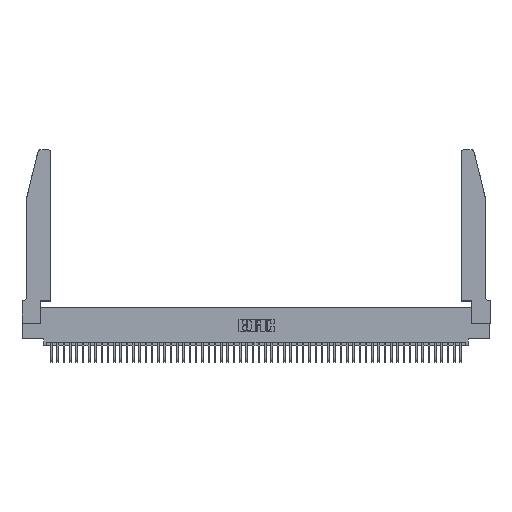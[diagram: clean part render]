
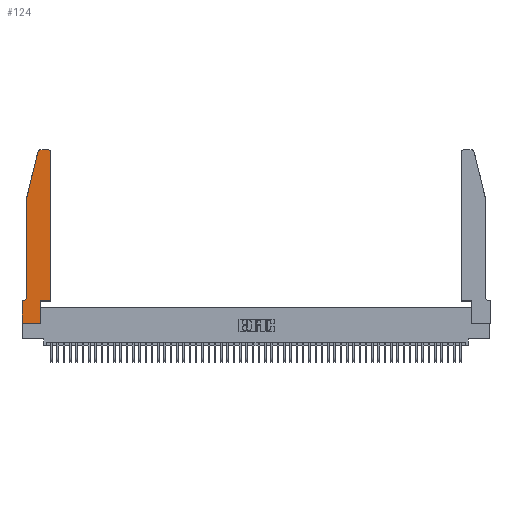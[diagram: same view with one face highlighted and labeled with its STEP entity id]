
A CAD part, top view. The second image highlights one B-rep face of the part: STEP entity #124.
In plain terms, the highlighted planar face has unit normal (0, 0, 1).
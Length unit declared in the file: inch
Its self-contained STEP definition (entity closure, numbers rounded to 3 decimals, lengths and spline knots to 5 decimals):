
#15 = ORIENTED_EDGE ( 'NONE', *, *, #23897, .T. ) ;
#124 = ADVANCED_FACE ( 'NONE', ( #39384 ), #39674, .T. ) ;
#1099 = DIRECTION ( 'NONE',  ( 0., 1., 0. ) ) ;
#1379 = ORIENTED_EDGE ( 'NONE', *, *, #29608, .T. ) ;
#2006 = VECTOR ( 'NONE', #28703, 39.37008 ) ;
#3244 = LINE ( 'NONE', #48450, #2006 ) ;
#4232 = CARTESIAN_POINT ( 'NONE',  ( 0.25487, 2.72718, 0.37 ) ) ;
#4593 = EDGE_CURVE ( 'NONE', #8375, #41574, #28886, .T. ) ;
#5065 = LINE ( 'NONE', #24567, #36732 ) ;
#5510 = LINE ( 'NONE', #48771, #25394 ) ;
#6583 = AXIS2_PLACEMENT_3D ( 'NONE', #27704, #43654, #19914 ) ;
#6850 = ORIENTED_EDGE ( 'NONE', *, *, #48446, .T. ) ;
#7034 = VECTOR ( 'NONE', #32559, 39.37008 ) ;
#7330 = DIRECTION ( 'NONE',  ( 0., 0., 1. ) ) ;
#8375 = VERTEX_POINT ( 'NONE', #35295 ) ;
#9034 = CARTESIAN_POINT ( 'NONE',  ( 0.4505, 2.72, 0.37 ) ) ;
#9817 = DIRECTION ( 'NONE',  ( 0., 0., 1. ) ) ;
#9950 = VERTEX_POINT ( 'NONE', #9034 ) ;
#10357 = AXIS2_PLACEMENT_3D ( 'NONE', #33581, #9817, #37562 ) ;
#10695 = CIRCLE ( 'NONE', #24376, 0.03 ) ;
#10829 = ORIENTED_EDGE ( 'NONE', *, *, #48861, .T. ) ;
#11004 = CARTESIAN_POINT ( 'NONE',  ( 0.284, 2.75, 0.37 ) ) ;
#12636 = CARTESIAN_POINT ( 'NONE',  ( 0., 0.35, 0.37 ) ) ;
#12967 = AXIS2_PLACEMENT_3D ( 'NONE', #16016, #43736, #19991 ) ;
#13276 = DIRECTION ( 'NONE',  ( -0.239, -0.971, 0. ) ) ;
#13375 = ORIENTED_EDGE ( 'NONE', *, *, #26790, .T. ) ;
#13861 = CARTESIAN_POINT ( 'NONE',  ( 0., 0., 0.37 ) ) ;
#13999 = DIRECTION ( 'NONE',  ( 0., 1., 0. ) ) ;
#15744 = EDGE_CURVE ( 'NONE', #19802, #9950, #48345, .T. ) ;
#15892 = EDGE_LOOP ( 'NONE', ( #45931, #6850, #15, #17568, #42987, #1379, #41827, #10829, #48661, #22004, #36300, #13375 ) ) ;
#16016 = CARTESIAN_POINT ( 'NONE',  ( 0.0055, 0.42, 0.37 ) ) ;
#16610 = CARTESIAN_POINT ( 'NONE',  ( 0.0755, 2., 0.37 ) ) ;
#17568 = ORIENTED_EDGE ( 'NONE', *, *, #4593, .T. ) ;
#17690 = VECTOR ( 'NONE', #33625, 39.37008 ) ;
#17998 = EDGE_CURVE ( 'NONE', #31756, #19168, #40022, .T. ) ;
#18228 = VERTEX_POINT ( 'NONE', #42941 ) ;
#18352 = VECTOR ( 'NONE', #48279, 39.37008 ) ;
#18448 = EDGE_CURVE ( 'NONE', #49311, #30130, #39975, .T. ) ;
#19012 = VECTOR ( 'NONE', #1099, 39.37008 ) ;
#19168 = VERTEX_POINT ( 'NONE', #24846 ) ;
#19802 = VERTEX_POINT ( 'NONE', #28429 ) ;
#19914 = DIRECTION ( 'NONE',  ( 1., 0., 0. ) ) ;
#19991 = DIRECTION ( 'NONE',  ( -1., 0., 0. ) ) ;
#22004 = ORIENTED_EDGE ( 'NONE', *, *, #50675, .T. ) ;
#23247 = CARTESIAN_POINT ( 'NONE',  ( 0.0755, 0.42, 0.37 ) ) ;
#23897 = EDGE_CURVE ( 'NONE', #25624, #8375, #5510, .T. ) ;
#24376 = AXIS2_PLACEMENT_3D ( 'NONE', #31119, #7330, #35089 ) ;
#24567 = CARTESIAN_POINT ( 'NONE',  ( 0.4505, 0.35, 0.37 ) ) ;
#24846 = CARTESIAN_POINT ( 'NONE',  ( 0., 0., 0.37 ) ) ;
#25394 = VECTOR ( 'NONE', #13276, 39.37008 ) ;
#25624 = VERTEX_POINT ( 'NONE', #4232 ) ;
#25761 = VERTEX_POINT ( 'NONE', #42844 ) ;
#26790 = EDGE_CURVE ( 'NONE', #9950, #49311, #42279, .T. ) ;
#27704 = CARTESIAN_POINT ( 'NONE',  ( 0., 0.35, 0.37 ) ) ;
#27706 = DIRECTION ( 'NONE',  ( -1., 0., 0. ) ) ;
#28429 = CARTESIAN_POINT ( 'NONE',  ( 0.4505, 0.35, 0.37 ) ) ;
#28540 = DIRECTION ( 'NONE',  ( 1., 0., 0. ) ) ;
#28703 = DIRECTION ( 'NONE',  ( 1., 0., 0. ) ) ;
#28886 = LINE ( 'NONE', #16610, #18352 ) ;
#29532 = LINE ( 'NONE', #36685, #19012 ) ;
#29608 = EDGE_CURVE ( 'NONE', #18228, #31756, #32767, .T. ) ;
#29754 = CARTESIAN_POINT ( 'NONE',  ( 0.4505, 0.35, 0.37 ) ) ;
#30130 = VERTEX_POINT ( 'NONE', #11004 ) ;
#31119 = CARTESIAN_POINT ( 'NONE',  ( 0.284, 2.72, 0.37 ) ) ;
#31270 = CARTESIAN_POINT ( 'NONE',  ( 0.4205, 2.75, 0.37 ) ) ;
#31509 = VECTOR ( 'NONE', #27706, 39.37008 ) ;
#31756 = VERTEX_POINT ( 'NONE', #12636 ) ;
#32559 = DIRECTION ( 'NONE',  ( -1., 0., 0. ) ) ;
#32767 = LINE ( 'NONE', #47263, #31509 ) ;
#33581 = CARTESIAN_POINT ( 'NONE',  ( 0.4205, 2.72, 0.37 ) ) ;
#33625 = DIRECTION ( 'NONE',  ( 0., -1., 0. ) ) ;
#35089 = DIRECTION ( 'NONE',  ( 1., 0., 0. ) ) ;
#35295 = CARTESIAN_POINT ( 'NONE',  ( 0.0755, 2., 0.37 ) ) ;
#36300 = ORIENTED_EDGE ( 'NONE', *, *, #15744, .T. ) ;
#36685 = CARTESIAN_POINT ( 'NONE',  ( 0.2865, 0.35, 0.37 ) ) ;
#36732 = VECTOR ( 'NONE', #28540, 39.37008 ) ;
#37562 = DIRECTION ( 'NONE',  ( 1., 0., 0. ) ) ;
#37807 = VECTOR ( 'NONE', #13999, 39.37008 ) ;
#39384 = FACE_OUTER_BOUND ( 'NONE', #15892, .T. ) ;
#39674 = PLANE ( 'NONE',  #6583 ) ;
#39975 = LINE ( 'NONE', #40355, #7034 ) ;
#40022 = LINE ( 'NONE', #13861, #17690 ) ;
#40355 = CARTESIAN_POINT ( 'NONE',  ( 0.2605, 2.75, 0.37 ) ) ;
#41574 = VERTEX_POINT ( 'NONE', #23247 ) ;
#41827 = ORIENTED_EDGE ( 'NONE', *, *, #17998, .T. ) ;
#42279 = CIRCLE ( 'NONE', #10357, 0.03 ) ;
#42844 = CARTESIAN_POINT ( 'NONE',  ( 0.2865, 0., 0.37 ) ) ;
#42941 = CARTESIAN_POINT ( 'NONE',  ( 0.0055, 0.35, 0.37 ) ) ;
#42987 = ORIENTED_EDGE ( 'NONE', *, *, #45750, .T. ) ;
#43654 = DIRECTION ( 'NONE',  ( 0., 0., 1. ) ) ;
#43736 = DIRECTION ( 'NONE',  ( 0., 0., -1. ) ) ;
#44962 = VERTEX_POINT ( 'NONE', #49987 ) ;
#45750 = EDGE_CURVE ( 'NONE', #41574, #18228, #46326, .T. ) ;
#45931 = ORIENTED_EDGE ( 'NONE', *, *, #18448, .T. ) ;
#46290 = EDGE_CURVE ( 'NONE', #25761, #44962, #29532, .T. ) ;
#46326 = CIRCLE ( 'NONE', #12967, 0.07 ) ;
#47263 = CARTESIAN_POINT ( 'NONE',  ( 0.0755, 0.35, 0.37 ) ) ;
#48279 = DIRECTION ( 'NONE',  ( 0., -1., 0. ) ) ;
#48345 = LINE ( 'NONE', #29754, #37807 ) ;
#48446 = EDGE_CURVE ( 'NONE', #30130, #25624, #10695, .T. ) ;
#48450 = CARTESIAN_POINT ( 'NONE',  ( 0., 0., 0.37 ) ) ;
#48661 = ORIENTED_EDGE ( 'NONE', *, *, #46290, .T. ) ;
#48771 = CARTESIAN_POINT ( 'NONE',  ( 0.0755, 2., 0.37 ) ) ;
#48861 = EDGE_CURVE ( 'NONE', #19168, #25761, #3244, .T. ) ;
#49311 = VERTEX_POINT ( 'NONE', #31270 ) ;
#49987 = CARTESIAN_POINT ( 'NONE',  ( 0.2865, 0.35, 0.37 ) ) ;
#50675 = EDGE_CURVE ( 'NONE', #44962, #19802, #5065, .T. ) ;
